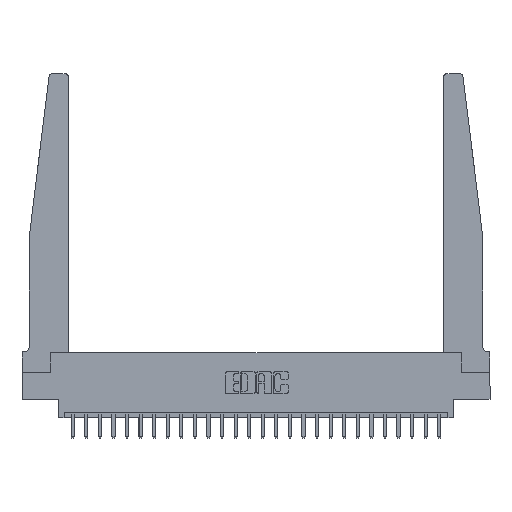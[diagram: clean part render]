
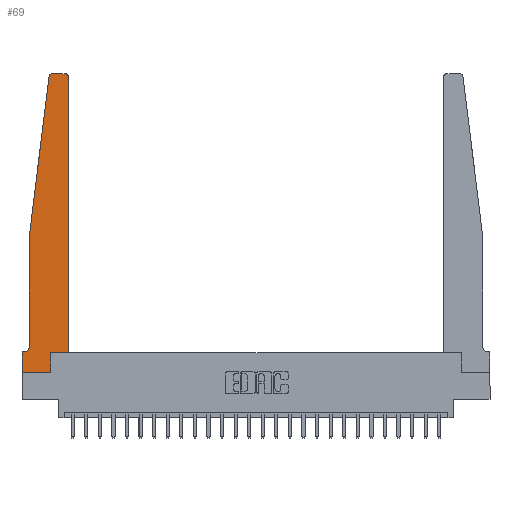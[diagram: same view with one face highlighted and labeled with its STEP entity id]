
A CAD part, top view. The second image highlights one B-rep face of the part: STEP entity #69.
In plain terms, the highlighted planar face has unit normal (0, 0, 1).
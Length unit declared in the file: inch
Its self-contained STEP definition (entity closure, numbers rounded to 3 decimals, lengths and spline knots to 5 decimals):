
#11 = ORIENTED_EDGE ( 'NONE', *, *, #21107, .T. ) ;
#16 = CARTESIAN_POINT ( 'NONE',  ( 0.015, 0.2375, 0.37 ) ) ;
#69 = ADVANCED_FACE ( 'NONE', ( #7122 ), #14917, .T. ) ;
#766 = VECTOR ( 'NONE', #24868, 39.37008 ) ;
#1128 = LINE ( 'NONE', #22250, #16182 ) ;
#1622 = CARTESIAN_POINT ( 'NONE',  ( 0.065, 0.1875, 0.37 ) ) ;
#1734 = VERTEX_POINT ( 'NONE', #21599 ) ;
#1780 = CARTESIAN_POINT ( 'NONE',  ( 0., 0., 0.37 ) ) ;
#2041 = DIRECTION ( 'NONE',  ( -1., 0., 0. ) ) ;
#2141 = CARTESIAN_POINT ( 'NONE',  ( 0., 0., 0.37 ) ) ;
#2143 = EDGE_CURVE ( 'NONE', #1734, #14551, #5760, .T. ) ;
#2204 = VECTOR ( 'NONE', #19527, 39.37008 ) ;
#3321 = DIRECTION ( 'NONE',  ( 1., 0., 0. ) ) ;
#3353 = DIRECTION ( 'NONE',  ( 0., 0., 1. ) ) ;
#3377 = CARTESIAN_POINT ( 'NONE',  ( 0.395, 2.72, 0.37 ) ) ;
#3812 = DIRECTION ( 'NONE',  ( 1., 0., 0. ) ) ;
#4209 = EDGE_CURVE ( 'NONE', #12816, #1734, #10239, .T. ) ;
#4211 = CARTESIAN_POINT ( 'NONE',  ( 0.27653, 2.72, 0.37 ) ) ;
#4508 = VERTEX_POINT ( 'NONE', #15356 ) ;
#4655 = LINE ( 'NONE', #1780, #15073 ) ;
#4758 = DIRECTION ( 'NONE',  ( 0., -1., 0. ) ) ;
#5343 = EDGE_CURVE ( 'NONE', #17084, #16325, #20774, .T. ) ;
#5760 = LINE ( 'NONE', #10609, #15519 ) ;
#5766 = EDGE_CURVE ( 'NONE', #20659, #10021, #12293, .T. ) ;
#6239 = DIRECTION ( 'NONE',  ( 1., 0., 0. ) ) ;
#6687 = VECTOR ( 'NONE', #17219, 39.37008 ) ;
#6846 = CARTESIAN_POINT ( 'NONE',  ( 0.27653, 2.75, 0.37 ) ) ;
#6899 = CIRCLE ( 'NONE', #8994, 0.03 ) ;
#6997 = DIRECTION ( 'NONE',  ( 0., 0., 1. ) ) ;
#7025 = DIRECTION ( 'NONE',  ( 1., 0., 0. ) ) ;
#7122 = FACE_OUTER_BOUND ( 'NONE', #17666, .T. ) ;
#7126 = VECTOR ( 'NONE', #19217, 39.37008 ) ;
#7665 = EDGE_CURVE ( 'NONE', #10021, #20499, #16961, .T. ) ;
#8127 = CARTESIAN_POINT ( 'NONE',  ( 0., 0.1875, 0.37 ) ) ;
#8475 = ORIENTED_EDGE ( 'NONE', *, *, #24205, .T. ) ;
#8655 = DIRECTION ( 'NONE',  ( -1., 0., 0. ) ) ;
#8994 = AXIS2_PLACEMENT_3D ( 'NONE', #4211, #17841, #6239 ) ;
#10021 = VERTEX_POINT ( 'NONE', #16205 ) ;
#10091 = ORIENTED_EDGE ( 'NONE', *, *, #25175, .T. ) ;
#10239 = CIRCLE ( 'NONE', #18442, 0.03 ) ;
#10266 = DIRECTION ( 'NONE',  ( 0., 1., 0. ) ) ;
#10277 = CARTESIAN_POINT ( 'NONE',  ( 0.065, 1.25, 0.37 ) ) ;
#10609 = CARTESIAN_POINT ( 'NONE',  ( 0.25, 2.75, 0.37 ) ) ;
#10612 = EDGE_CURVE ( 'NONE', #20499, #19488, #4655, .T. ) ;
#10921 = ORIENTED_EDGE ( 'NONE', *, *, #7665, .T. ) ;
#12293 = LINE ( 'NONE', #1622, #7126 ) ;
#12709 = EDGE_CURVE ( 'NONE', #16325, #4508, #1128, .T. ) ;
#12816 = VERTEX_POINT ( 'NONE', #12977 ) ;
#12977 = CARTESIAN_POINT ( 'NONE',  ( 0.425, 2.72, 0.37 ) ) ;
#13857 = DIRECTION ( 'NONE',  ( 0., 0., -1. ) ) ;
#14212 = DIRECTION ( 'NONE',  ( -0.122, -0.992, 0. ) ) ;
#14329 = CARTESIAN_POINT ( 'NONE',  ( 0.2605, 0., 0.37 ) ) ;
#14551 = VERTEX_POINT ( 'NONE', #6846 ) ;
#14917 = PLANE ( 'NONE',  #23858 ) ;
#15073 = VECTOR ( 'NONE', #3812, 39.37008 ) ;
#15356 = CARTESIAN_POINT ( 'NONE',  ( 0.065, 0.2375, 0.37 ) ) ;
#15519 = VECTOR ( 'NONE', #8655, 39.37008 ) ;
#15533 = ORIENTED_EDGE ( 'NONE', *, *, #12709, .T. ) ;
#15893 = VECTOR ( 'NONE', #10266, 39.37008 ) ;
#16007 = EDGE_CURVE ( 'NONE', #4508, #20659, #16616, .T. ) ;
#16182 = VECTOR ( 'NONE', #4758, 39.37008 ) ;
#16205 = CARTESIAN_POINT ( 'NONE',  ( 0., 0.1875, 0.37 ) ) ;
#16325 = VERTEX_POINT ( 'NONE', #21521 ) ;
#16616 = CIRCLE ( 'NONE', #24055, 0.05 ) ;
#16876 = CARTESIAN_POINT ( 'NONE',  ( 0.425, 0.18, 0.37 ) ) ;
#16961 = LINE ( 'NONE', #21044, #6687 ) ;
#17084 = VERTEX_POINT ( 'NONE', #24193 ) ;
#17219 = DIRECTION ( 'NONE',  ( 0., -1., 0. ) ) ;
#17326 = ORIENTED_EDGE ( 'NONE', *, *, #5343, .T. ) ;
#17666 = EDGE_LOOP ( 'NONE', ( #21222, #22314, #17326, #15533, #21868, #17863, #10921, #19208, #11, #10091, #8475, #19839 ) ) ;
#17791 = LINE ( 'NONE', #23415, #2204 ) ;
#17841 = DIRECTION ( 'NONE',  ( 0., 0., 1. ) ) ;
#17863 = ORIENTED_EDGE ( 'NONE', *, *, #5766, .T. ) ;
#17891 = CARTESIAN_POINT ( 'NONE',  ( 0.2605, 0.18, 0.37 ) ) ;
#18273 = CARTESIAN_POINT ( 'NONE',  ( 0.015, 0.1875, 0.37 ) ) ;
#18442 = AXIS2_PLACEMENT_3D ( 'NONE', #3377, #3353, #3321 ) ;
#19208 = ORIENTED_EDGE ( 'NONE', *, *, #10612, .T. ) ;
#19217 = DIRECTION ( 'NONE',  ( -1., 0., 0. ) ) ;
#19488 = VERTEX_POINT ( 'NONE', #14329 ) ;
#19527 = DIRECTION ( 'NONE',  ( 0., 1., 0. ) ) ;
#19839 = ORIENTED_EDGE ( 'NONE', *, *, #4209, .T. ) ;
#19884 = CARTESIAN_POINT ( 'NONE',  ( 0.425, 0.18, 0.37 ) ) ;
#20133 = VERTEX_POINT ( 'NONE', #17891 ) ;
#20342 = LINE ( 'NONE', #23022, #766 ) ;
#20499 = VERTEX_POINT ( 'NONE', #2141 ) ;
#20659 = VERTEX_POINT ( 'NONE', #18273 ) ;
#20774 = LINE ( 'NONE', #10277, #22572 ) ;
#21018 = LINE ( 'NONE', #19884, #15893 ) ;
#21044 = CARTESIAN_POINT ( 'NONE',  ( 0., 0., 0.37 ) ) ;
#21107 = EDGE_CURVE ( 'NONE', #19488, #20133, #17791, .T. ) ;
#21173 = EDGE_CURVE ( 'NONE', #14551, #17084, #6899, .T. ) ;
#21222 = ORIENTED_EDGE ( 'NONE', *, *, #2143, .T. ) ;
#21521 = CARTESIAN_POINT ( 'NONE',  ( 0.065, 1.25, 0.37 ) ) ;
#21581 = VERTEX_POINT ( 'NONE', #16876 ) ;
#21599 = CARTESIAN_POINT ( 'NONE',  ( 0.395, 2.75, 0.37 ) ) ;
#21868 = ORIENTED_EDGE ( 'NONE', *, *, #16007, .T. ) ;
#22250 = CARTESIAN_POINT ( 'NONE',  ( 0.065, 1.25, 0.37 ) ) ;
#22314 = ORIENTED_EDGE ( 'NONE', *, *, #21173, .T. ) ;
#22572 = VECTOR ( 'NONE', #14212, 39.37008 ) ;
#23022 = CARTESIAN_POINT ( 'NONE',  ( 0.425, 0.18, 0.37 ) ) ;
#23415 = CARTESIAN_POINT ( 'NONE',  ( 0.2605, 0.18, 0.37 ) ) ;
#23858 = AXIS2_PLACEMENT_3D ( 'NONE', #8127, #6997, #7025 ) ;
#24055 = AXIS2_PLACEMENT_3D ( 'NONE', #16, #13857, #2041 ) ;
#24193 = CARTESIAN_POINT ( 'NONE',  ( 0.24675, 2.72367, 0.37 ) ) ;
#24205 = EDGE_CURVE ( 'NONE', #21581, #12816, #21018, .T. ) ;
#24868 = DIRECTION ( 'NONE',  ( 1., 0., 0. ) ) ;
#25175 = EDGE_CURVE ( 'NONE', #20133, #21581, #20342, .T. ) ;
